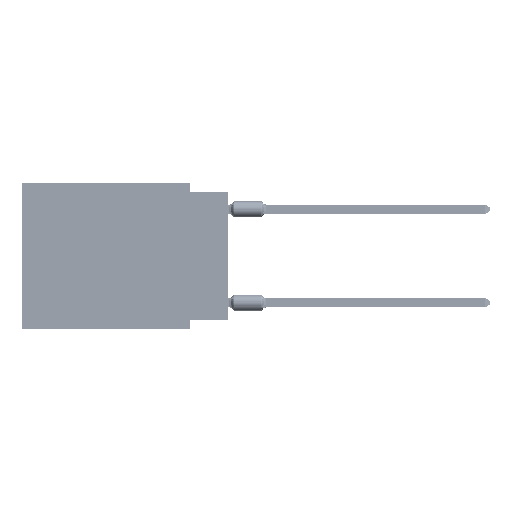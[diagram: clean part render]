
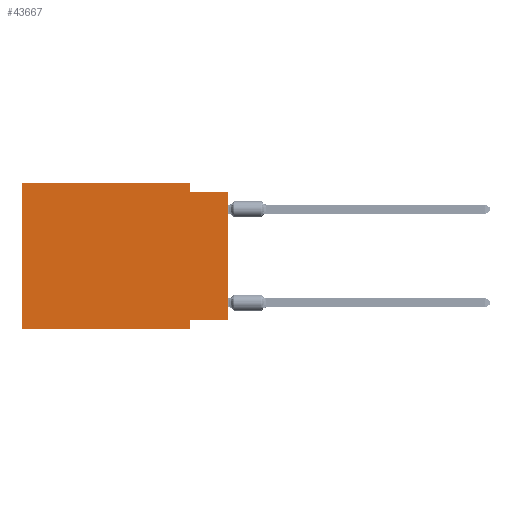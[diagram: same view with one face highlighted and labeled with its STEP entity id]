
A CAD part, left-side view. The second image highlights one B-rep face of the part: STEP entity #43667.
In plain terms, the highlighted planar face has unit normal (-1, 0, 0).
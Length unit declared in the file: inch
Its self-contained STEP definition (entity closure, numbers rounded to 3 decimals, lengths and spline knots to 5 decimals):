
#1075 = CARTESIAN_POINT ( 'NONE',  ( 0., 0.1, -0.39 ) ) ;
#1394 = LINE ( 'NONE', #56098, #13481 ) ;
#2332 = VECTOR ( 'NONE', #87420, 39.37008 ) ;
#3780 = DIRECTION ( 'NONE',  ( 0., 1., 0. ) ) ;
#4738 = ORIENTED_EDGE ( 'NONE', *, *, #44358, .F. ) ;
#5686 = ORIENTED_EDGE ( 'NONE', *, *, #78661, .F. ) ;
#7500 = ORIENTED_EDGE ( 'NONE', *, *, #78314, .T. ) ;
#7772 = CARTESIAN_POINT ( 'NONE',  ( 0., 0.55, 0. ) ) ;
#8935 = VECTOR ( 'NONE', #8968, 39.37008 ) ;
#8968 = DIRECTION ( 'NONE',  ( 0., 0., -1. ) ) ;
#10383 = VECTOR ( 'NONE', #70586, 39.37008 ) ;
#13278 = LINE ( 'NONE', #7772, #74151 ) ;
#13481 = VECTOR ( 'NONE', #57433, 39.37008 ) ;
#13967 = CARTESIAN_POINT ( 'NONE',  ( 0., 0.1, -0.365 ) ) ;
#14905 = LINE ( 'NONE', #49979, #8935 ) ;
#16147 = EDGE_LOOP ( 'NONE', ( #56783, #25266, #5686, #4738, #62962, #7500, #58602, #75123 ) ) ;
#16534 = VERTEX_POINT ( 'NONE', #51645 ) ;
#17895 = CARTESIAN_POINT ( 'NONE',  ( 0., 0., -0.365 ) ) ;
#20850 = CARTESIAN_POINT ( 'NONE',  ( 0., 0., -0.365 ) ) ;
#21352 = VERTEX_POINT ( 'NONE', #1075 ) ;
#21673 = EDGE_CURVE ( 'NONE', #16534, #60597, #87605, .T. ) ;
#24077 = EDGE_CURVE ( 'NONE', #89851, #65887, #60696, .T. ) ;
#25266 = ORIENTED_EDGE ( 'NONE', *, *, #31582, .F. ) ;
#28140 = VERTEX_POINT ( 'NONE', #73583 ) ;
#28927 = CARTESIAN_POINT ( 'NONE',  ( 0., 0.55, 0. ) ) ;
#31582 = EDGE_CURVE ( 'NONE', #64412, #28140, #85653, .T. ) ;
#31853 = LINE ( 'NONE', #59626, #2332 ) ;
#34026 = CARTESIAN_POINT ( 'NONE',  ( 0., 0.1, -0.025 ) ) ;
#38051 = PLANE ( 'NONE',  #82737 ) ;
#40868 = VECTOR ( 'NONE', #45562, 39.37008 ) ;
#41951 = DIRECTION ( 'NONE',  ( 0., -1., 0. ) ) ;
#42806 = CARTESIAN_POINT ( 'NONE',  ( 0., 0.55, -0.39 ) ) ;
#43667 = ADVANCED_FACE ( 'NONE', ( #72668 ), #38051, .F. ) ;
#44358 = EDGE_CURVE ( 'NONE', #60597, #70298, #13278, .T. ) ;
#44528 = VECTOR ( 'NONE', #3780, 39.37008 ) ;
#45562 = DIRECTION ( 'NONE',  ( 0., -1., 0. ) ) ;
#49979 = CARTESIAN_POINT ( 'NONE',  ( 0., 0.1, 0. ) ) ;
#50376 = EDGE_CURVE ( 'NONE', #65887, #21352, #1394, .T. ) ;
#51645 = CARTESIAN_POINT ( 'NONE',  ( 0., 0.55, -0.39 ) ) ;
#53875 = CARTESIAN_POINT ( 'NONE',  ( 0., 0.55, 0. ) ) ;
#56098 = CARTESIAN_POINT ( 'NONE',  ( 0., 0.1, -0.39 ) ) ;
#56783 = ORIENTED_EDGE ( 'NONE', *, *, #70179, .T. ) ;
#57417 = VECTOR ( 'NONE', #81646, 39.37008 ) ;
#57433 = DIRECTION ( 'NONE',  ( 0., 0., -1. ) ) ;
#58327 = CARTESIAN_POINT ( 'NONE',  ( 0., 0., -0.025 ) ) ;
#58602 = ORIENTED_EDGE ( 'NONE', *, *, #50376, .F. ) ;
#59626 = CARTESIAN_POINT ( 'NONE',  ( 0., 0., 0. ) ) ;
#60597 = VERTEX_POINT ( 'NONE', #28927 ) ;
#60696 = LINE ( 'NONE', #17895, #44528 ) ;
#62962 = ORIENTED_EDGE ( 'NONE', *, *, #21673, .F. ) ;
#64412 = VERTEX_POINT ( 'NONE', #34026 ) ;
#64928 = CARTESIAN_POINT ( 'NONE',  ( 0., 0.55, 0. ) ) ;
#65841 = DIRECTION ( 'NONE',  ( 0., 0., -1. ) ) ;
#65887 = VERTEX_POINT ( 'NONE', #13967 ) ;
#68708 = CARTESIAN_POINT ( 'NONE',  ( 0., 0.1, 0. ) ) ;
#70179 = EDGE_CURVE ( 'NONE', #89851, #28140, #31853, .T. ) ;
#70298 = VERTEX_POINT ( 'NONE', #68708 ) ;
#70586 = DIRECTION ( 'NONE',  ( 0., -1., 0. ) ) ;
#72668 = FACE_OUTER_BOUND ( 'NONE', #16147, .T. ) ;
#73583 = CARTESIAN_POINT ( 'NONE',  ( 0., 0., -0.025 ) ) ;
#74151 = VECTOR ( 'NONE', #41951, 39.37008 ) ;
#75123 = ORIENTED_EDGE ( 'NONE', *, *, #24077, .F. ) ;
#77414 = LINE ( 'NONE', #42806, #10383 ) ;
#78314 = EDGE_CURVE ( 'NONE', #16534, #21352, #77414, .T. ) ;
#78661 = EDGE_CURVE ( 'NONE', #70298, #64412, #14905, .T. ) ;
#80396 = DIRECTION ( 'NONE',  ( 1., 0., 0. ) ) ;
#81646 = DIRECTION ( 'NONE',  ( 0., 0., 1. ) ) ;
#82737 = AXIS2_PLACEMENT_3D ( 'NONE', #64928, #80396, #65841 ) ;
#85653 = LINE ( 'NONE', #58327, #40868 ) ;
#87420 = DIRECTION ( 'NONE',  ( 0., 0., 1. ) ) ;
#87605 = LINE ( 'NONE', #53875, #57417 ) ;
#89851 = VERTEX_POINT ( 'NONE', #20850 ) ;
